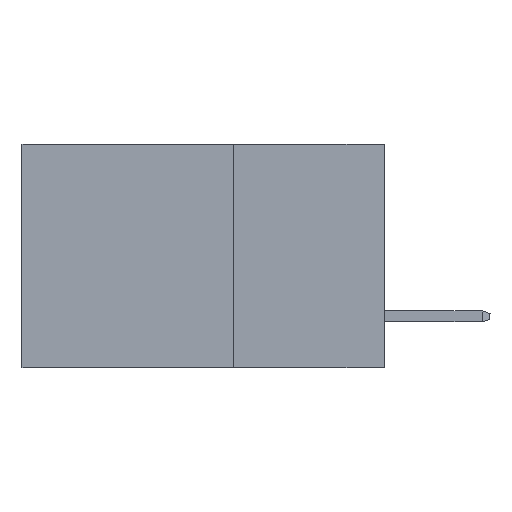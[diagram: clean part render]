
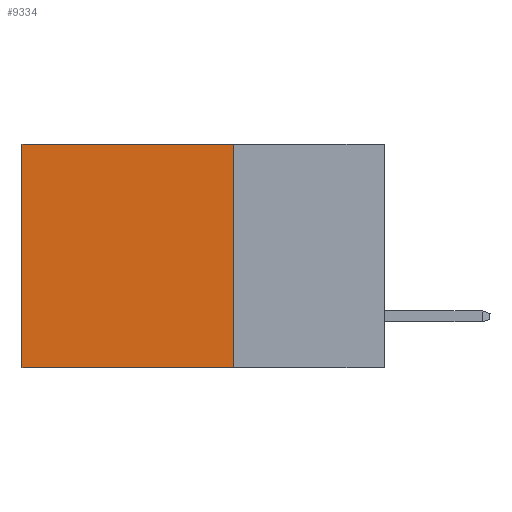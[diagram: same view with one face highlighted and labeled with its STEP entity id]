
A CAD part, left-side view. The second image highlights one B-rep face of the part: STEP entity #9334.
In plain terms, the highlighted planar face has unit normal (-1, 0, 0).
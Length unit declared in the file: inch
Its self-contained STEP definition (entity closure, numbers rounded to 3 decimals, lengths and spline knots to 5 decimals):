
#67 = CARTESIAN_POINT ( 'NONE',  ( 0.2615, 0.25, 0. ) ) ;
#110 = DIRECTION ( 'NONE',  ( 0., 1., 0. ) ) ;
#175 = VECTOR ( 'NONE', #110, 39.37008 ) ;
#1090 = VECTOR ( 'NONE', #8644, 39.37008 ) ;
#1474 = LINE ( 'NONE', #5404, #1090 ) ;
#2087 = ORIENTED_EDGE ( 'NONE', *, *, #3005, .F. ) ;
#2505 = LINE ( 'NONE', #5593, #175 ) ;
#3005 = EDGE_CURVE ( 'NONE', #9057, #9254, #3196, .T. ) ;
#3196 = LINE ( 'NONE', #6361, #6642 ) ;
#3563 = DIRECTION ( 'NONE',  ( 0., 0., -1. ) ) ;
#3664 = AXIS2_PLACEMENT_3D ( 'NONE', #9119, #8432, #3563 ) ;
#4184 = CARTESIAN_POINT ( 'NONE',  ( 0.2615, 0.25, -0.37 ) ) ;
#5269 = EDGE_LOOP ( 'NONE', ( #7665, #7881, #2087, #8781 ) ) ;
#5404 = CARTESIAN_POINT ( 'NONE',  ( 0.2615, 0.25, 0. ) ) ;
#5412 = VERTEX_POINT ( 'NONE', #10230 ) ;
#5520 = EDGE_CURVE ( 'NONE', #8573, #5412, #6417, .T. ) ;
#5593 = CARTESIAN_POINT ( 'NONE',  ( 0.2615, 0.25, -0.37 ) ) ;
#5634 = VECTOR ( 'NONE', #6270, 39.37008 ) ;
#6050 = CARTESIAN_POINT ( 'NONE',  ( 0.2615, 0.6, 0. ) ) ;
#6170 = DIRECTION ( 'NONE',  ( 0., 0., -1. ) ) ;
#6270 = DIRECTION ( 'NONE',  ( 0., 0., -1. ) ) ;
#6361 = CARTESIAN_POINT ( 'NONE',  ( 0.2615, 0.25, -0.37 ) ) ;
#6417 = LINE ( 'NONE', #7211, #5634 ) ;
#6642 = VECTOR ( 'NONE', #6170, 39.37008 ) ;
#6684 = PLANE ( 'NONE',  #3664 ) ;
#6741 = EDGE_CURVE ( 'NONE', #9254, #5412, #2505, .T. ) ;
#7211 = CARTESIAN_POINT ( 'NONE',  ( 0.2615, 0.6, -0.37 ) ) ;
#7665 = ORIENTED_EDGE ( 'NONE', *, *, #5520, .T. ) ;
#7787 = EDGE_CURVE ( 'NONE', #9057, #8573, #1474, .T. ) ;
#7881 = ORIENTED_EDGE ( 'NONE', *, *, #6741, .F. ) ;
#8432 = DIRECTION ( 'NONE',  ( 1., 0., 0. ) ) ;
#8573 = VERTEX_POINT ( 'NONE', #6050 ) ;
#8644 = DIRECTION ( 'NONE',  ( 0., 1., 0. ) ) ;
#8781 = ORIENTED_EDGE ( 'NONE', *, *, #7787, .T. ) ;
#9057 = VERTEX_POINT ( 'NONE', #67 ) ;
#9119 = CARTESIAN_POINT ( 'NONE',  ( 0.2615, 0.25, -0.37 ) ) ;
#9254 = VERTEX_POINT ( 'NONE', #4184 ) ;
#9334 = ADVANCED_FACE ( 'NONE', ( #10012 ), #6684, .F. ) ;
#10012 = FACE_OUTER_BOUND ( 'NONE', #5269, .T. ) ;
#10230 = CARTESIAN_POINT ( 'NONE',  ( 0.2615, 0.6, -0.37 ) ) ;
